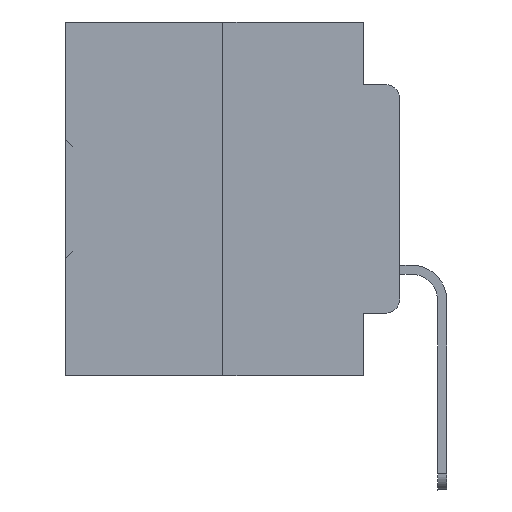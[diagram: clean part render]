
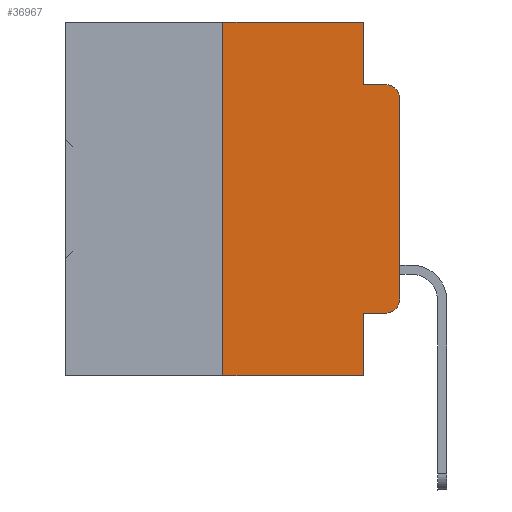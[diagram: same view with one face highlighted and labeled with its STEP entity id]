
A CAD part, left-side view. The second image highlights one B-rep face of the part: STEP entity #36967.
In plain terms, the highlighted planar face has unit normal (-1, 0, 0).
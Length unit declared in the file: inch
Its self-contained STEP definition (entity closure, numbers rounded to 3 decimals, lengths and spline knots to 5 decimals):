
#9 = VERTEX_POINT ( 'NONE', #31535 ) ;
#378 = CARTESIAN_POINT ( 'NONE',  ( 0., 0.051, -0.4115 ) ) ;
#1494 = CIRCLE ( 'NONE', #9382, 0.02 ) ;
#1907 = ORIENTED_EDGE ( 'NONE', *, *, #7309, .T. ) ;
#2415 = LINE ( 'NONE', #2988, #26429 ) ;
#2743 = VECTOR ( 'NONE', #25498, 39.37008 ) ;
#2988 = CARTESIAN_POINT ( 'NONE',  ( 0., 0., 0. ) ) ;
#2994 = CARTESIAN_POINT ( 'NONE',  ( 0., 0.051, -0.0885 ) ) ;
#3844 = EDGE_LOOP ( 'NONE', ( #1907, #19263, #4909, #26339, #20404, #30708, #21645, #6535, #14534, #21497 ) ) ;
#4909 = ORIENTED_EDGE ( 'NONE', *, *, #35084, .F. ) ;
#5879 = VECTOR ( 'NONE', #22435, 39.37008 ) ;
#6170 = CARTESIAN_POINT ( 'NONE',  ( 0., 0.25, 0. ) ) ;
#6426 = EDGE_CURVE ( 'NONE', #26168, #16678, #1494, .T. ) ;
#6535 = ORIENTED_EDGE ( 'NONE', *, *, #7679, .F. ) ;
#6737 = CARTESIAN_POINT ( 'NONE',  ( 0., 0.473, 0. ) ) ;
#7309 = EDGE_CURVE ( 'NONE', #16678, #34803, #2415, .T. ) ;
#7679 = EDGE_CURVE ( 'NONE', #9, #31703, #22473, .T. ) ;
#8210 = EDGE_CURVE ( 'NONE', #34803, #33090, #18568, .T. ) ;
#8846 = VECTOR ( 'NONE', #11304, 39.37008 ) ;
#9286 = DIRECTION ( 'NONE',  ( 0., -1., 0. ) ) ;
#9382 = AXIS2_PLACEMENT_3D ( 'NONE', #17711, #12031, #9874 ) ;
#9874 = DIRECTION ( 'NONE',  ( 0., 0., -1. ) ) ;
#10310 = PLANE ( 'NONE',  #34267 ) ;
#10476 = CARTESIAN_POINT ( 'NONE',  ( 0., 0.473, -0.5 ) ) ;
#11220 = LINE ( 'NONE', #378, #35360 ) ;
#11292 = EDGE_CURVE ( 'NONE', #25299, #30571, #25509, .T. ) ;
#11304 = DIRECTION ( 'NONE',  ( 0., 0., -1. ) ) ;
#11678 = VECTOR ( 'NONE', #9286, 39.37008 ) ;
#11957 = LINE ( 'NONE', #26218, #11678 ) ;
#12031 = DIRECTION ( 'NONE',  ( -1., 0., 0. ) ) ;
#12163 = CARTESIAN_POINT ( 'NONE',  ( 0., 0.02, -0.1085 ) ) ;
#12299 = VERTEX_POINT ( 'NONE', #6170 ) ;
#13936 = CARTESIAN_POINT ( 'NONE',  ( 0., 0.051, 0. ) ) ;
#13981 = DIRECTION ( 'NONE',  ( 0., 0., 1. ) ) ;
#14534 = ORIENTED_EDGE ( 'NONE', *, *, #24102, .T. ) ;
#16285 = LINE ( 'NONE', #21795, #17986 ) ;
#16678 = VERTEX_POINT ( 'NONE', #17486 ) ;
#17486 = CARTESIAN_POINT ( 'NONE',  ( 0., 0., -0.3915 ) ) ;
#17711 = CARTESIAN_POINT ( 'NONE',  ( 0., 0.02, -0.3915 ) ) ;
#17824 = CARTESIAN_POINT ( 'NONE',  ( 0., 0.02, -0.0885 ) ) ;
#17986 = VECTOR ( 'NONE', #37008, 39.37008 ) ;
#18504 = FACE_OUTER_BOUND ( 'NONE', #3844, .T. ) ;
#18568 = CIRCLE ( 'NONE', #24075, 0.02 ) ;
#19178 = CARTESIAN_POINT ( 'NONE',  ( 0., 0.051, -0.5 ) ) ;
#19263 = ORIENTED_EDGE ( 'NONE', *, *, #8210, .T. ) ;
#20404 = ORIENTED_EDGE ( 'NONE', *, *, #30001, .F. ) ;
#21497 = ORIENTED_EDGE ( 'NONE', *, *, #6426, .T. ) ;
#21645 = ORIENTED_EDGE ( 'NONE', *, *, #29993, .T. ) ;
#21795 = CARTESIAN_POINT ( 'NONE',  ( 0., 0.25, 0. ) ) ;
#21863 = LINE ( 'NONE', #10476, #2743 ) ;
#22435 = DIRECTION ( 'NONE',  ( 0., 0., -1. ) ) ;
#22473 = LINE ( 'NONE', #13936, #8846 ) ;
#22756 = VERTEX_POINT ( 'NONE', #36881 ) ;
#24075 = AXIS2_PLACEMENT_3D ( 'NONE', #12163, #32334, #26998 ) ;
#24102 = EDGE_CURVE ( 'NONE', #9, #26168, #11220, .T. ) ;
#24754 = DIRECTION ( 'NONE',  ( 0., -1., 0. ) ) ;
#25299 = VERTEX_POINT ( 'NONE', #34788 ) ;
#25498 = DIRECTION ( 'NONE',  ( 0., -1., 0. ) ) ;
#25509 = LINE ( 'NONE', #27957, #5879 ) ;
#26168 = VERTEX_POINT ( 'NONE', #29850 ) ;
#26218 = CARTESIAN_POINT ( 'NONE',  ( 0., 0.051, -0.0885 ) ) ;
#26339 = ORIENTED_EDGE ( 'NONE', *, *, #11292, .F. ) ;
#26429 = VECTOR ( 'NONE', #13981, 39.37008 ) ;
#26998 = DIRECTION ( 'NONE',  ( 0., 0., -1. ) ) ;
#27957 = CARTESIAN_POINT ( 'NONE',  ( 0., 0.051, 0. ) ) ;
#28694 = DIRECTION ( 'NONE',  ( 0., -1., 0. ) ) ;
#29850 = CARTESIAN_POINT ( 'NONE',  ( 0., 0.02, -0.4115 ) ) ;
#29993 = EDGE_CURVE ( 'NONE', #22756, #31703, #21863, .T. ) ;
#30001 = EDGE_CURVE ( 'NONE', #12299, #25299, #30644, .T. ) ;
#30121 = DIRECTION ( 'NONE',  ( 0., 0., -1. ) ) ;
#30407 = CARTESIAN_POINT ( 'NONE',  ( 0., 0., -0.1085 ) ) ;
#30571 = VERTEX_POINT ( 'NONE', #2994 ) ;
#30644 = LINE ( 'NONE', #36717, #37322 ) ;
#30708 = ORIENTED_EDGE ( 'NONE', *, *, #33423, .F. ) ;
#31535 = CARTESIAN_POINT ( 'NONE',  ( 0., 0.051, -0.4115 ) ) ;
#31703 = VERTEX_POINT ( 'NONE', #19178 ) ;
#32334 = DIRECTION ( 'NONE',  ( -1., 0., 0. ) ) ;
#32781 = DIRECTION ( 'NONE',  ( 1., 0., 0. ) ) ;
#33090 = VERTEX_POINT ( 'NONE', #17824 ) ;
#33423 = EDGE_CURVE ( 'NONE', #22756, #12299, #16285, .T. ) ;
#34267 = AXIS2_PLACEMENT_3D ( 'NONE', #6737, #32781, #30121 ) ;
#34788 = CARTESIAN_POINT ( 'NONE',  ( 0., 0.051, 0. ) ) ;
#34803 = VERTEX_POINT ( 'NONE', #30407 ) ;
#35084 = EDGE_CURVE ( 'NONE', #30571, #33090, #11957, .T. ) ;
#35360 = VECTOR ( 'NONE', #28694, 39.37008 ) ;
#36717 = CARTESIAN_POINT ( 'NONE',  ( 0., 0.473, 0. ) ) ;
#36881 = CARTESIAN_POINT ( 'NONE',  ( 0., 0.25, -0.5 ) ) ;
#36967 = ADVANCED_FACE ( 'NONE', ( #18504 ), #10310, .F. ) ;
#37008 = DIRECTION ( 'NONE',  ( 0., 0., 1. ) ) ;
#37322 = VECTOR ( 'NONE', #24754, 39.37008 ) ;
